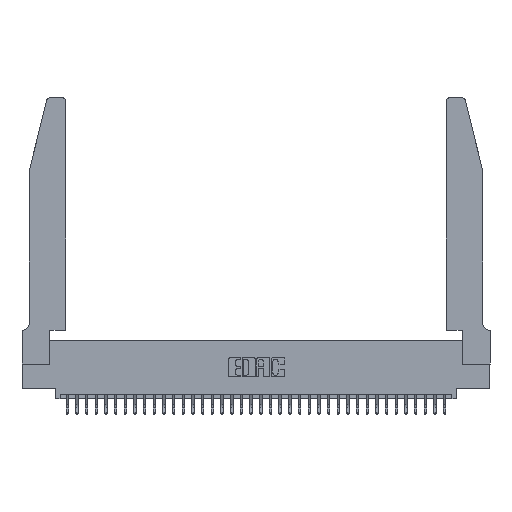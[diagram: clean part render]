
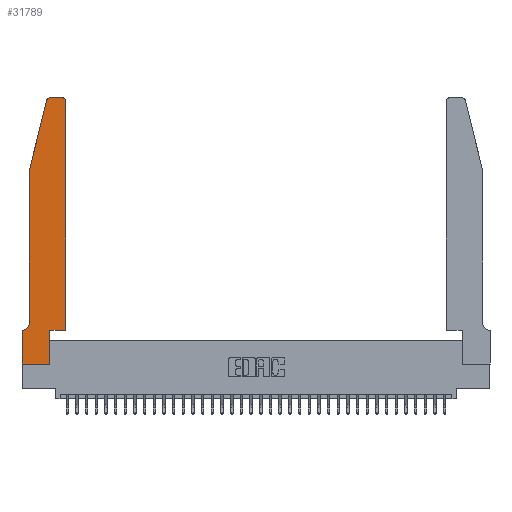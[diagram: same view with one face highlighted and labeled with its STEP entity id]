
A CAD part, top view. The second image highlights one B-rep face of the part: STEP entity #31789.
In plain terms, the highlighted planar face has unit normal (0, 0, 1).
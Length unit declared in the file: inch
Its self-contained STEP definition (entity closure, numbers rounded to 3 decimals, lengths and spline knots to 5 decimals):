
#41 = LINE ( 'NONE', #10179, #10739 ) ;
#343 = CIRCLE ( 'NONE', #18320, 0.03 ) ;
#913 = VECTOR ( 'NONE', #9051, 39.37008 ) ;
#933 = EDGE_CURVE ( 'NONE', #23566, #3767, #2893, .T. ) ;
#1718 = DIRECTION ( 'NONE',  ( 0., 0., 1. ) ) ;
#2025 = AXIS2_PLACEMENT_3D ( 'NONE', #7981, #27612, #4967 ) ;
#2208 = CIRCLE ( 'NONE', #25904, 0.07 ) ;
#2792 = DIRECTION ( 'NONE',  ( -1., 0., 0. ) ) ;
#2893 = LINE ( 'NONE', #28058, #25629 ) ;
#3714 = VERTEX_POINT ( 'NONE', #35420 ) ;
#3767 = VERTEX_POINT ( 'NONE', #22095 ) ;
#3889 = EDGE_CURVE ( 'NONE', #19439, #6564, #41, .T. ) ;
#4067 = LINE ( 'NONE', #20703, #913 ) ;
#4083 = CARTESIAN_POINT ( 'NONE',  ( 0.2865, 0., 0.37 ) ) ;
#4387 = LINE ( 'NONE', #13056, #26232 ) ;
#4589 = DIRECTION ( 'NONE',  ( -1., 0., 0. ) ) ;
#4644 = DIRECTION ( 'NONE',  ( 0., 0., 1. ) ) ;
#4769 = CARTESIAN_POINT ( 'NONE',  ( 0.4505, 2.72, 0.37 ) ) ;
#4774 = EDGE_CURVE ( 'NONE', #22298, #5095, #4387, .T. ) ;
#4967 = DIRECTION ( 'NONE',  ( 1., 0., 0. ) ) ;
#4987 = DIRECTION ( 'NONE',  ( 0., 1., 0. ) ) ;
#5095 = VERTEX_POINT ( 'NONE', #4769 ) ;
#5188 = EDGE_CURVE ( 'NONE', #5095, #3714, #343, .T. ) ;
#6068 = FACE_OUTER_BOUND ( 'NONE', #21416, .T. ) ;
#6366 = CARTESIAN_POINT ( 'NONE',  ( 0.0055, 0.35, 0.37 ) ) ;
#6564 = VERTEX_POINT ( 'NONE', #4083 ) ;
#6665 = LINE ( 'NONE', #22033, #16988 ) ;
#6967 = CARTESIAN_POINT ( 'NONE',  ( 0.0755, 2., 0.37 ) ) ;
#7072 = DIRECTION ( 'NONE',  ( 0., 0., -1. ) ) ;
#7975 = LINE ( 'NONE', #10449, #34174 ) ;
#7981 = CARTESIAN_POINT ( 'NONE',  ( 0., 0.35, 0.37 ) ) ;
#8188 = AXIS2_PLACEMENT_3D ( 'NONE', #32715, #4644, #35928 ) ;
#8342 = CARTESIAN_POINT ( 'NONE',  ( 0.2865, 0.35, 0.37 ) ) ;
#8935 = EDGE_CURVE ( 'NONE', #3767, #19439, #23939, .T. ) ;
#9042 = EDGE_CURVE ( 'NONE', #3714, #15536, #7975, .T. ) ;
#9051 = DIRECTION ( 'NONE',  ( -0.239, -0.971, 0. ) ) ;
#9695 = VECTOR ( 'NONE', #30058, 39.37008 ) ;
#10179 = CARTESIAN_POINT ( 'NONE',  ( 0., 0., 0.37 ) ) ;
#10449 = CARTESIAN_POINT ( 'NONE',  ( 0.2605, 2.75, 0.37 ) ) ;
#10739 = VECTOR ( 'NONE', #22009, 39.37008 ) ;
#12739 = VERTEX_POINT ( 'NONE', #13894 ) ;
#13023 = CIRCLE ( 'NONE', #8188, 0.03 ) ;
#13056 = CARTESIAN_POINT ( 'NONE',  ( 0.4505, 0.35, 0.37 ) ) ;
#13325 = DIRECTION ( 'NONE',  ( 0., 1., 0. ) ) ;
#13338 = EDGE_CURVE ( 'NONE', #6564, #31993, #6665, .T. ) ;
#13378 = ORIENTED_EDGE ( 'NONE', *, *, #3889, .T. ) ;
#13894 = CARTESIAN_POINT ( 'NONE',  ( 0.0755, 0.42, 0.37 ) ) ;
#13937 = EDGE_CURVE ( 'NONE', #12739, #23566, #2208, .T. ) ;
#14165 = CARTESIAN_POINT ( 'NONE',  ( 0.4505, 0.35, 0.37 ) ) ;
#15536 = VERTEX_POINT ( 'NONE', #19132 ) ;
#15812 = VECTOR ( 'NONE', #30754, 39.37008 ) ;
#16241 = ORIENTED_EDGE ( 'NONE', *, *, #22021, .T. ) ;
#16327 = DIRECTION ( 'NONE',  ( -1., 0., 0. ) ) ;
#16988 = VECTOR ( 'NONE', #4987, 39.37008 ) ;
#18022 = ORIENTED_EDGE ( 'NONE', *, *, #26407, .T. ) ;
#18320 = AXIS2_PLACEMENT_3D ( 'NONE', #24543, #1718, #24678 ) ;
#18751 = CARTESIAN_POINT ( 'NONE',  ( 0., 0., 0.37 ) ) ;
#18774 = CARTESIAN_POINT ( 'NONE',  ( 0.0055, 0.42, 0.37 ) ) ;
#19054 = CARTESIAN_POINT ( 'NONE',  ( 0.4505, 0.35, 0.37 ) ) ;
#19132 = CARTESIAN_POINT ( 'NONE',  ( 0.284, 2.75, 0.37 ) ) ;
#19439 = VERTEX_POINT ( 'NONE', #22728 ) ;
#20703 = CARTESIAN_POINT ( 'NONE',  ( 0.0755, 2., 0.37 ) ) ;
#21314 = ORIENTED_EDGE ( 'NONE', *, *, #33414, .T. ) ;
#21416 = EDGE_LOOP ( 'NONE', ( #30531, #16241, #21314, #28227, #22294, #29170, #24562, #13378, #24510, #18022, #25945, #33695 ) ) ;
#22009 = DIRECTION ( 'NONE',  ( 1., 0., 0. ) ) ;
#22021 = EDGE_CURVE ( 'NONE', #15536, #32642, #13023, .T. ) ;
#22033 = CARTESIAN_POINT ( 'NONE',  ( 0.2865, 0.35, 0.37 ) ) ;
#22095 = CARTESIAN_POINT ( 'NONE',  ( 0., 0.35, 0.37 ) ) ;
#22294 = ORIENTED_EDGE ( 'NONE', *, *, #13937, .T. ) ;
#22298 = VERTEX_POINT ( 'NONE', #14165 ) ;
#22728 = CARTESIAN_POINT ( 'NONE',  ( 0., 0., 0.37 ) ) ;
#23566 = VERTEX_POINT ( 'NONE', #6366 ) ;
#23939 = LINE ( 'NONE', #18751, #9695 ) ;
#24510 = ORIENTED_EDGE ( 'NONE', *, *, #13338, .T. ) ;
#24543 = CARTESIAN_POINT ( 'NONE',  ( 0.4205, 2.72, 0.37 ) ) ;
#24562 = ORIENTED_EDGE ( 'NONE', *, *, #8935, .T. ) ;
#24678 = DIRECTION ( 'NONE',  ( 1., 0., 0. ) ) ;
#25042 = PLANE ( 'NONE',  #2025 ) ;
#25145 = CARTESIAN_POINT ( 'NONE',  ( 0.0755, 2., 0.37 ) ) ;
#25230 = LINE ( 'NONE', #19054, #15812 ) ;
#25334 = LINE ( 'NONE', #25145, #27033 ) ;
#25629 = VECTOR ( 'NONE', #2792, 39.37008 ) ;
#25904 = AXIS2_PLACEMENT_3D ( 'NONE', #18774, #7072, #4589 ) ;
#25945 = ORIENTED_EDGE ( 'NONE', *, *, #4774, .T. ) ;
#26232 = VECTOR ( 'NONE', #13325, 39.37008 ) ;
#26407 = EDGE_CURVE ( 'NONE', #31993, #22298, #25230, .T. ) ;
#27033 = VECTOR ( 'NONE', #30814, 39.37008 ) ;
#27612 = DIRECTION ( 'NONE',  ( 0., 0., 1. ) ) ;
#28058 = CARTESIAN_POINT ( 'NONE',  ( 0.0755, 0.35, 0.37 ) ) ;
#28227 = ORIENTED_EDGE ( 'NONE', *, *, #35583, .T. ) ;
#28557 = VERTEX_POINT ( 'NONE', #6967 ) ;
#29170 = ORIENTED_EDGE ( 'NONE', *, *, #933, .T. ) ;
#29268 = CARTESIAN_POINT ( 'NONE',  ( 0.25487, 2.72718, 0.37 ) ) ;
#30058 = DIRECTION ( 'NONE',  ( 0., -1., 0. ) ) ;
#30531 = ORIENTED_EDGE ( 'NONE', *, *, #9042, .T. ) ;
#30754 = DIRECTION ( 'NONE',  ( 1., 0., 0. ) ) ;
#30814 = DIRECTION ( 'NONE',  ( 0., -1., 0. ) ) ;
#31789 = ADVANCED_FACE ( 'NONE', ( #6068 ), #25042, .T. ) ;
#31993 = VERTEX_POINT ( 'NONE', #8342 ) ;
#32642 = VERTEX_POINT ( 'NONE', #29268 ) ;
#32715 = CARTESIAN_POINT ( 'NONE',  ( 0.284, 2.72, 0.37 ) ) ;
#33414 = EDGE_CURVE ( 'NONE', #32642, #28557, #4067, .T. ) ;
#33695 = ORIENTED_EDGE ( 'NONE', *, *, #5188, .T. ) ;
#34174 = VECTOR ( 'NONE', #16327, 39.37008 ) ;
#35420 = CARTESIAN_POINT ( 'NONE',  ( 0.4205, 2.75, 0.37 ) ) ;
#35583 = EDGE_CURVE ( 'NONE', #28557, #12739, #25334, .T. ) ;
#35928 = DIRECTION ( 'NONE',  ( 1., 0., 0. ) ) ;
